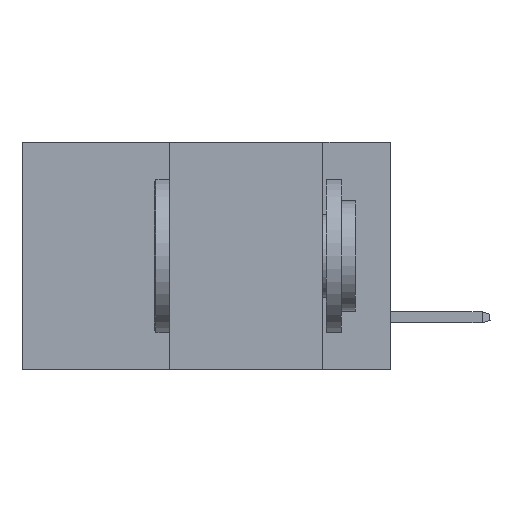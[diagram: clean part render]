
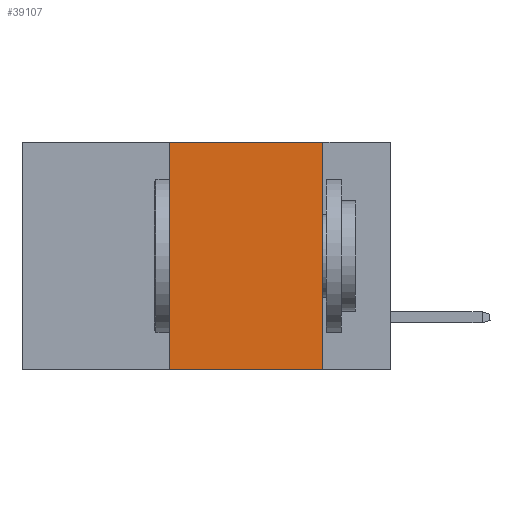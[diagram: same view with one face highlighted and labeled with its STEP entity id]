
A CAD part, left-side view. The second image highlights one B-rep face of the part: STEP entity #39107.
In plain terms, the highlighted planar face has unit normal (-1, 0, 0).
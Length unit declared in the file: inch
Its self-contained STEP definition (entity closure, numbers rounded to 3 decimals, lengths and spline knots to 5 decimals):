
#563 = VERTEX_POINT ( 'NONE', #39695 ) ;
#962 = DIRECTION ( 'NONE',  ( 0., -1., 0. ) ) ;
#5768 = CARTESIAN_POINT ( 'NONE',  ( 0., 0.11, 0. ) ) ;
#6262 = VECTOR ( 'NONE', #16800, 39.37008 ) ;
#6632 = VECTOR ( 'NONE', #962, 39.37008 ) ;
#7381 = PLANE ( 'NONE',  #40674 ) ;
#7738 = LINE ( 'NONE', #8100, #6632 ) ;
#8100 = CARTESIAN_POINT ( 'NONE',  ( 0., 0.6, 0. ) ) ;
#8368 = LINE ( 'NONE', #20477, #28137 ) ;
#9269 = DIRECTION ( 'NONE',  ( 0., -1., 0. ) ) ;
#11413 = LINE ( 'NONE', #5768, #6262 ) ;
#13698 = DIRECTION ( 'NONE',  ( 0., 0., 1. ) ) ;
#16800 = DIRECTION ( 'NONE',  ( 0., 0., -1. ) ) ;
#18015 = ORIENTED_EDGE ( 'NONE', *, *, #36706, .T. ) ;
#18235 = ORIENTED_EDGE ( 'NONE', *, *, #29332, .F. ) ;
#19354 = CARTESIAN_POINT ( 'NONE',  ( 0., 0.11, 0. ) ) ;
#20477 = CARTESIAN_POINT ( 'NONE',  ( 0., 0.6, -0.37 ) ) ;
#22590 = CARTESIAN_POINT ( 'NONE',  ( 0., 0.6, 0. ) ) ;
#22858 = VECTOR ( 'NONE', #13698, 39.37008 ) ;
#24625 = LINE ( 'NONE', #26578, #22858 ) ;
#25234 = CARTESIAN_POINT ( 'NONE',  ( 0., 0.36, 0. ) ) ;
#26578 = CARTESIAN_POINT ( 'NONE',  ( 0., 0.36, 0. ) ) ;
#28137 = VECTOR ( 'NONE', #9269, 39.37008 ) ;
#28791 = ORIENTED_EDGE ( 'NONE', *, *, #28826, .F. ) ;
#28826 = EDGE_CURVE ( 'NONE', #563, #42658, #24625, .T. ) ;
#29332 = EDGE_CURVE ( 'NONE', #42658, #37850, #7738, .T. ) ;
#29999 = DIRECTION ( 'NONE',  ( 1., 0., 0. ) ) ;
#31360 = FACE_OUTER_BOUND ( 'NONE', #44011, .T. ) ;
#31703 = CARTESIAN_POINT ( 'NONE',  ( 0., 0.11, -0.37 ) ) ;
#32592 = ORIENTED_EDGE ( 'NONE', *, *, #46676, .F. ) ;
#33587 = VERTEX_POINT ( 'NONE', #31703 ) ;
#36706 = EDGE_CURVE ( 'NONE', #563, #33587, #8368, .T. ) ;
#37850 = VERTEX_POINT ( 'NONE', #19354 ) ;
#39107 = ADVANCED_FACE ( 'NONE', ( #31360 ), #7381, .F. ) ;
#39695 = CARTESIAN_POINT ( 'NONE',  ( 0., 0.36, -0.37 ) ) ;
#40674 = AXIS2_PLACEMENT_3D ( 'NONE', #22590, #29999, #44260 ) ;
#42658 = VERTEX_POINT ( 'NONE', #25234 ) ;
#44011 = EDGE_LOOP ( 'NONE', ( #32592, #18235, #28791, #18015 ) ) ;
#44260 = DIRECTION ( 'NONE',  ( 0., 0., -1. ) ) ;
#46676 = EDGE_CURVE ( 'NONE', #37850, #33587, #11413, .T. ) ;
